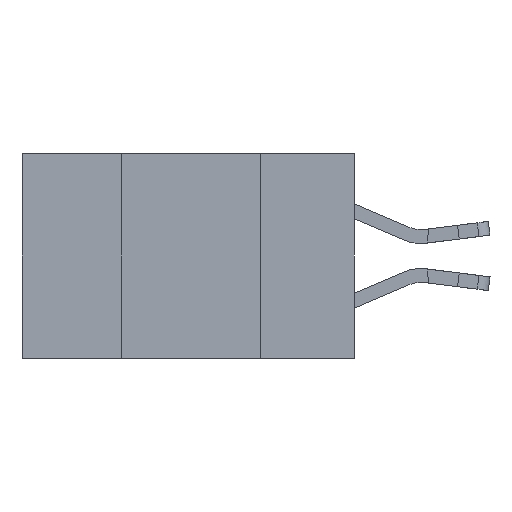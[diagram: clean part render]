
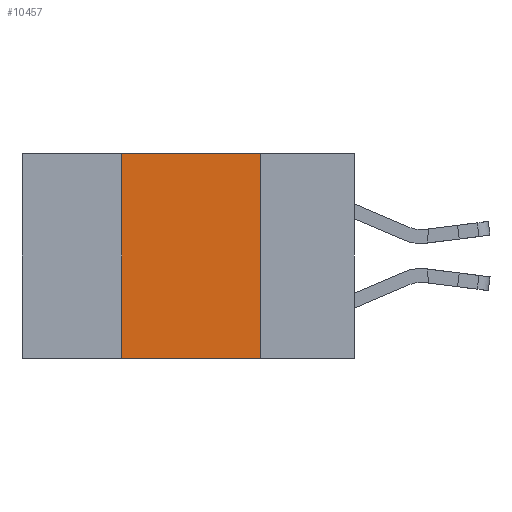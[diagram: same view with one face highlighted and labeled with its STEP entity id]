
A CAD part, left-side view. The second image highlights one B-rep face of the part: STEP entity #10457.
In plain terms, the highlighted planar face has unit normal (-1, 0, 0).
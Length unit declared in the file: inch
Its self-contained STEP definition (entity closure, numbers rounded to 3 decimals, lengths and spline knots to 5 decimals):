
#1956 = LINE ( 'NONE', #10991, #11316 ) ;
#1966 = VECTOR ( 'NONE', #12978, 39.37008 ) ;
#3490 = FACE_OUTER_BOUND ( 'NONE', #9201, .T. ) ;
#4863 = CARTESIAN_POINT ( 'NONE',  ( 0., 0.6, -0.37 ) ) ;
#5204 = LINE ( 'NONE', #13060, #1966 ) ;
#5516 = VERTEX_POINT ( 'NONE', #12015 ) ;
#5801 = CARTESIAN_POINT ( 'NONE',  ( 0., 0.42, -0.37 ) ) ;
#5920 = ORIENTED_EDGE ( 'NONE', *, *, #14438, .T. ) ;
#5950 = ORIENTED_EDGE ( 'NONE', *, *, #15397, .F. ) ;
#6713 = CARTESIAN_POINT ( 'NONE',  ( 0., 0.42, 0. ) ) ;
#6888 = DIRECTION ( 'NONE',  ( 0., 0., -1. ) ) ;
#6906 = DIRECTION ( 'NONE',  ( 1., 0., 0. ) ) ;
#6916 = AXIS2_PLACEMENT_3D ( 'NONE', #6923, #6906, #6888 ) ;
#6923 = CARTESIAN_POINT ( 'NONE',  ( 0., 0.6, 0. ) ) ;
#6958 = PLANE ( 'NONE',  #6916 ) ;
#7031 = DIRECTION ( 'NONE',  ( 0., 0., 1. ) ) ;
#7653 = ORIENTED_EDGE ( 'NONE', *, *, #7694, .F. ) ;
#7655 = CARTESIAN_POINT ( 'NONE',  ( 0., 0.42, -0.37 ) ) ;
#7694 = EDGE_CURVE ( 'NONE', #14047, #5516, #1956, .T. ) ;
#9201 = EDGE_LOOP ( 'NONE', ( #7653, #11622, #5950, #5920 ) ) ;
#9624 = EDGE_CURVE ( 'NONE', #14114, #14047, #5204, .T. ) ;
#9755 = VECTOR ( 'NONE', #7031, 39.37008 ) ;
#10263 = CARTESIAN_POINT ( 'NONE',  ( 0., 0.17, 0. ) ) ;
#10457 = ADVANCED_FACE ( 'NONE', ( #3490 ), #6958, .F. ) ;
#10991 = CARTESIAN_POINT ( 'NONE',  ( 0., 0.17, -0.37 ) ) ;
#11316 = VECTOR ( 'NONE', #11411, 39.37008 ) ;
#11411 = DIRECTION ( 'NONE',  ( 0., 0., -1. ) ) ;
#11622 = ORIENTED_EDGE ( 'NONE', *, *, #9624, .F. ) ;
#12015 = CARTESIAN_POINT ( 'NONE',  ( 0., 0.17, -0.37 ) ) ;
#12172 = DIRECTION ( 'NONE',  ( 0., -1., 0. ) ) ;
#12978 = DIRECTION ( 'NONE',  ( 0., -1., 0. ) ) ;
#13060 = CARTESIAN_POINT ( 'NONE',  ( 0., 0.6, 0. ) ) ;
#13372 = LINE ( 'NONE', #5801, #9755 ) ;
#14047 = VERTEX_POINT ( 'NONE', #10263 ) ;
#14114 = VERTEX_POINT ( 'NONE', #6713 ) ;
#14438 = EDGE_CURVE ( 'NONE', #14513, #5516, #15579, .T. ) ;
#14513 = VERTEX_POINT ( 'NONE', #7655 ) ;
#14859 = VECTOR ( 'NONE', #12172, 39.37008 ) ;
#15397 = EDGE_CURVE ( 'NONE', #14513, #14114, #13372, .T. ) ;
#15579 = LINE ( 'NONE', #4863, #14859 ) ;
